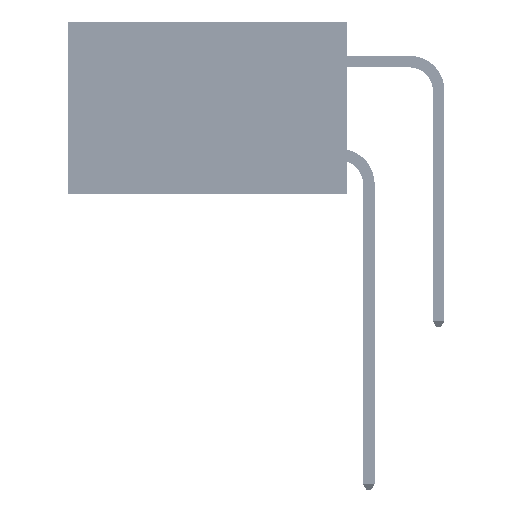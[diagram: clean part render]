
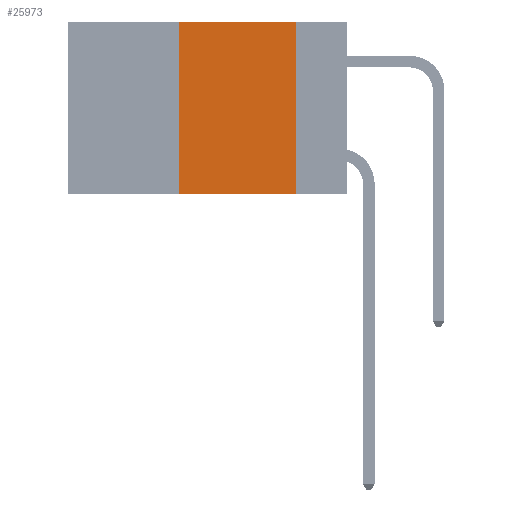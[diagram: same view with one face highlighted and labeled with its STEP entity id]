
A CAD part, left-side view. The second image highlights one B-rep face of the part: STEP entity #25973.
In plain terms, the highlighted planar face has unit normal (-1, 0, 0).
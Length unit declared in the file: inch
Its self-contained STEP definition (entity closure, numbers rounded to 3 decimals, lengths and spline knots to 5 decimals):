
#1644 = DIRECTION ( 'NONE',  ( 0., 0., -1. ) ) ;
#3894 = PLANE ( 'NONE',  #51163 ) ;
#9445 = EDGE_CURVE ( 'NONE', #9567, #15650, #31789, .T. ) ;
#9450 = CARTESIAN_POINT ( 'NONE',  ( 0., 0.36, 0. ) ) ;
#9567 = VERTEX_POINT ( 'NONE', #30463 ) ;
#11595 = ORIENTED_EDGE ( 'NONE', *, *, #35814, .F. ) ;
#12469 = DIRECTION ( 'NONE',  ( 0., 0., -1. ) ) ;
#13157 = EDGE_CURVE ( 'NONE', #9567, #14439, #20283, .T. ) ;
#14299 = DIRECTION ( 'NONE',  ( 0., -1., 0. ) ) ;
#14439 = VERTEX_POINT ( 'NONE', #35713 ) ;
#14909 = FACE_OUTER_BOUND ( 'NONE', #24686, .T. ) ;
#15233 = VECTOR ( 'NONE', #52101, 39.37008 ) ;
#15650 = VERTEX_POINT ( 'NONE', #9450 ) ;
#17202 = VECTOR ( 'NONE', #20580, 39.37008 ) ;
#17805 = LINE ( 'NONE', #45072, #17202 ) ;
#20283 = LINE ( 'NONE', #50855, #49706 ) ;
#20580 = DIRECTION ( 'NONE',  ( 0., -1., 0. ) ) ;
#20615 = DIRECTION ( 'NONE',  ( 1., 0., 0. ) ) ;
#21975 = CARTESIAN_POINT ( 'NONE',  ( 0., 0.6, 0. ) ) ;
#24686 = EDGE_LOOP ( 'NONE', ( #41025, #11595, #50042, #48772 ) ) ;
#25973 = ADVANCED_FACE ( 'NONE', ( #14909 ), #3894, .F. ) ;
#26764 = EDGE_CURVE ( 'NONE', #32256, #14439, #44138, .T. ) ;
#28325 = CARTESIAN_POINT ( 'NONE',  ( 0., 0.36, 0. ) ) ;
#30463 = CARTESIAN_POINT ( 'NONE',  ( 0., 0.36, -0.37 ) ) ;
#31789 = LINE ( 'NONE', #28325, #15233 ) ;
#32256 = VERTEX_POINT ( 'NONE', #43292 ) ;
#35713 = CARTESIAN_POINT ( 'NONE',  ( 0., 0.11, -0.37 ) ) ;
#35814 = EDGE_CURVE ( 'NONE', #15650, #32256, #17805, .T. ) ;
#38377 = VECTOR ( 'NONE', #1644, 39.37008 ) ;
#38395 = CARTESIAN_POINT ( 'NONE',  ( 0., 0.11, 0. ) ) ;
#41025 = ORIENTED_EDGE ( 'NONE', *, *, #26764, .F. ) ;
#43292 = CARTESIAN_POINT ( 'NONE',  ( 0., 0.11, 0. ) ) ;
#44138 = LINE ( 'NONE', #38395, #38377 ) ;
#45072 = CARTESIAN_POINT ( 'NONE',  ( 0., 0.6, 0. ) ) ;
#48772 = ORIENTED_EDGE ( 'NONE', *, *, #13157, .T. ) ;
#49706 = VECTOR ( 'NONE', #14299, 39.37008 ) ;
#50042 = ORIENTED_EDGE ( 'NONE', *, *, #9445, .F. ) ;
#50855 = CARTESIAN_POINT ( 'NONE',  ( 0., 0.6, -0.37 ) ) ;
#51163 = AXIS2_PLACEMENT_3D ( 'NONE', #21975, #20615, #12469 ) ;
#52101 = DIRECTION ( 'NONE',  ( 0., 0., 1. ) ) ;
